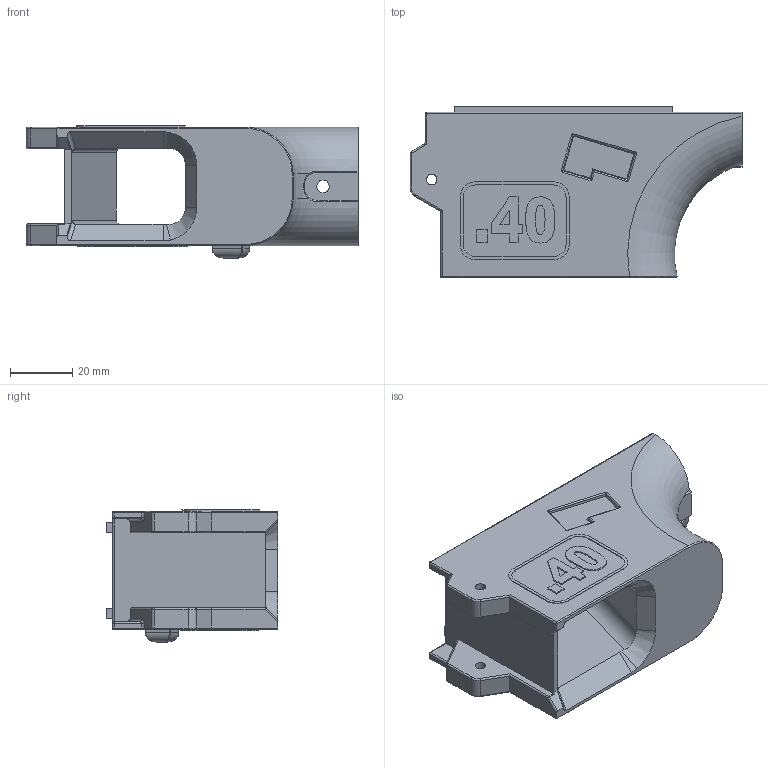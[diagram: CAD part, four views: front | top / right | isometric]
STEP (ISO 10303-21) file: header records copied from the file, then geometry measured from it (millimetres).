
FILE_DESCRIPTION(/* description */ (''),/* implementation_level */ '2;1');
FILE_NAME(/* name */ '40 cal MagWell GLOCK MAGS.stp',/* time_stamp */ '2020-07-05T03:18:57+03:00',/* author */ (''),/* organization */ (''),/* preprocessor_version */ 'ST-DEVELOPER v15.2',/* originating_system */ 'Autodesk Translator Framework v2.0.0.5431',/* authorisation */ '');
FILE_SCHEMA (('AUTOMOTIVE_DESIGN { 1 0 10303 214 3 1 1 }'));
Length unit declared in the file: centimetre
Products named in the file (1): 40SW
Bounding box: 106.51 x 55 x 42.4 mm (x, y, z)
Volume: 113278.7 mm3; surface area: 31297.5 mm2
Topology: 10 solids, 10 shells, 465 faces, 1191 edges, 736 vertices
Faces by surface type: plane 181, bspline 129, cylinder 127, torus 16, sphere 10, cone 2
Full cylindrical faces by diameter (mm): 1.5 x2, 3.4 x2, 4 x2
Entity records: 17081 total; most frequent: CARTESIAN_POINT 6427, ORIENTED_EDGE 2344, DIRECTION 1935, EDGE_CURVE 1172, VERTEX_POINT 735, LINE 677, VECTOR 677, AXIS2_PLACEMENT_3D 629
